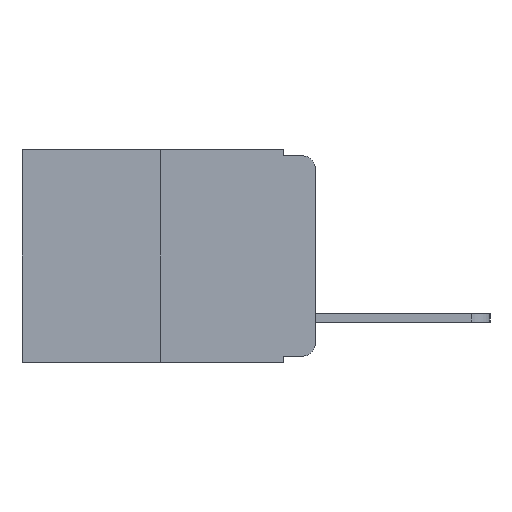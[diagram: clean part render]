
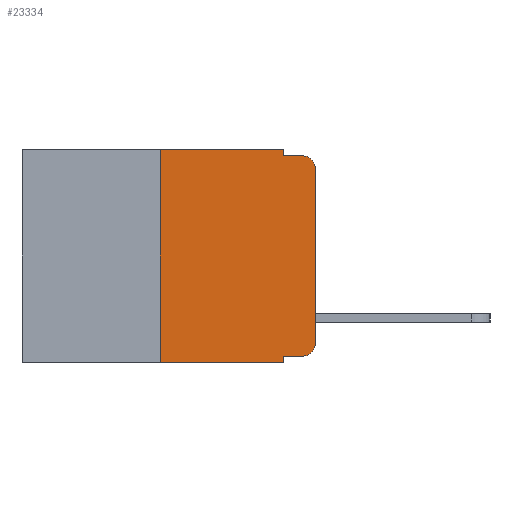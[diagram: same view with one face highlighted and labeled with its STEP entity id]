
A CAD part, left-side view. The second image highlights one B-rep face of the part: STEP entity #23334.
In plain terms, the highlighted planar face has unit normal (-1, 0, 0).
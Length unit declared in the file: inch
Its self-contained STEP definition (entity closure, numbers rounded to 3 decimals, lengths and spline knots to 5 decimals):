
#84 = EDGE_CURVE ( 'NONE', #15799, #23277, #23887, .T. ) ;
#361 = DIRECTION ( 'NONE',  ( 0., 0., -1. ) ) ;
#553 = EDGE_CURVE ( 'NONE', #23277, #15689, #18922, .T. ) ;
#712 = DIRECTION ( 'NONE',  ( 0., -1., 0. ) ) ;
#917 = VERTEX_POINT ( 'NONE', #17587 ) ;
#1067 = DIRECTION ( 'NONE',  ( 0., 0., -1. ) ) ;
#1223 = DIRECTION ( 'NONE',  ( 0., 0., -1. ) ) ;
#2070 = CARTESIAN_POINT ( 'NONE',  ( 0., 0., -0.03 ) ) ;
#2336 = EDGE_CURVE ( 'NONE', #12085, #21058, #13135, .T. ) ;
#2639 = DIRECTION ( 'NONE',  ( -1., 0., 0. ) ) ;
#3029 = CARTESIAN_POINT ( 'NONE',  ( 0., 0.02, -0.313 ) ) ;
#3619 = LINE ( 'NONE', #4112, #12368 ) ;
#4039 = VECTOR ( 'NONE', #19675, 39.37008 ) ;
#4112 = CARTESIAN_POINT ( 'NONE',  ( 0., 0.473, -0.343 ) ) ;
#4740 = VECTOR ( 'NONE', #361, 39.37008 ) ;
#4872 = ORIENTED_EDGE ( 'NONE', *, *, #553, .F. ) ;
#5501 = LINE ( 'NONE', #16483, #14811 ) ;
#6026 = ORIENTED_EDGE ( 'NONE', *, *, #84, .F. ) ;
#6773 = CARTESIAN_POINT ( 'NONE',  ( 0., 0., 0. ) ) ;
#7125 = CARTESIAN_POINT ( 'NONE',  ( 0., 0.02, -0.333 ) ) ;
#7201 = ORIENTED_EDGE ( 'NONE', *, *, #12765, .F. ) ;
#7516 = AXIS2_PLACEMENT_3D ( 'NONE', #23308, #12297, #1067 ) ;
#8140 = CARTESIAN_POINT ( 'NONE',  ( 0., 0.051, -0.01 ) ) ;
#8145 = LINE ( 'NONE', #6773, #17988 ) ;
#8295 = CARTESIAN_POINT ( 'NONE',  ( 0., 0.051, -0.333 ) ) ;
#8583 = CARTESIAN_POINT ( 'NONE',  ( 0., 0.051, 0. ) ) ;
#8944 = DIRECTION ( 'NONE',  ( 0., 0., -1. ) ) ;
#8949 = EDGE_CURVE ( 'NONE', #17417, #12085, #10854, .T. ) ;
#9150 = VECTOR ( 'NONE', #19411, 39.37008 ) ;
#9307 = CARTESIAN_POINT ( 'NONE',  ( 0., 0.051, 0. ) ) ;
#10078 = AXIS2_PLACEMENT_3D ( 'NONE', #3029, #2639, #8944 ) ;
#10107 = ORIENTED_EDGE ( 'NONE', *, *, #21632, .F. ) ;
#10854 = LINE ( 'NONE', #8295, #15743 ) ;
#11007 = DIRECTION ( 'NONE',  ( 0., 0., 1. ) ) ;
#11079 = VERTEX_POINT ( 'NONE', #14723 ) ;
#11113 = VERTEX_POINT ( 'NONE', #2070 ) ;
#11368 = EDGE_CURVE ( 'NONE', #11113, #11079, #21504, .T. ) ;
#11538 = EDGE_LOOP ( 'NONE', ( #20494, #11862, #13038, #4872, #6026, #7201, #18777, #10107, #13610, #12443 ) ) ;
#11862 = ORIENTED_EDGE ( 'NONE', *, *, #11368, .T. ) ;
#12040 = CARTESIAN_POINT ( 'NONE',  ( 0., 0.051, -0.01 ) ) ;
#12085 = VERTEX_POINT ( 'NONE', #7125 ) ;
#12297 = DIRECTION ( 'NONE',  ( -1., 0., 0. ) ) ;
#12368 = VECTOR ( 'NONE', #13474, 39.37008 ) ;
#12426 = DIRECTION ( 'NONE',  ( 1., 0., 0. ) ) ;
#12443 = ORIENTED_EDGE ( 'NONE', *, *, #2336, .T. ) ;
#12765 = EDGE_CURVE ( 'NONE', #17175, #15799, #5501, .T. ) ;
#13038 = ORIENTED_EDGE ( 'NONE', *, *, #16761, .F. ) ;
#13135 = CIRCLE ( 'NONE', #10078, 0.02 ) ;
#13474 = DIRECTION ( 'NONE',  ( 0., -1., 0. ) ) ;
#13610 = ORIENTED_EDGE ( 'NONE', *, *, #8949, .T. ) ;
#13879 = CARTESIAN_POINT ( 'NONE',  ( 0., 0.473, 0. ) ) ;
#14187 = PLANE ( 'NONE',  #20688 ) ;
#14723 = CARTESIAN_POINT ( 'NONE',  ( 0., 0.02, -0.01 ) ) ;
#14811 = VECTOR ( 'NONE', #11007, 39.37008 ) ;
#15689 = VERTEX_POINT ( 'NONE', #12040 ) ;
#15743 = VECTOR ( 'NONE', #21246, 39.37008 ) ;
#15799 = VERTEX_POINT ( 'NONE', #23302 ) ;
#15949 = CARTESIAN_POINT ( 'NONE',  ( 0., 0.473, 0. ) ) ;
#16483 = CARTESIAN_POINT ( 'NONE',  ( 0., 0.25, 0. ) ) ;
#16761 = EDGE_CURVE ( 'NONE', #15689, #11079, #22107, .T. ) ;
#17160 = FACE_OUTER_BOUND ( 'NONE', #11538, .T. ) ;
#17175 = VERTEX_POINT ( 'NONE', #22303 ) ;
#17412 = CARTESIAN_POINT ( 'NONE',  ( 0., 0.051, -0.333 ) ) ;
#17417 = VERTEX_POINT ( 'NONE', #17412 ) ;
#17587 = CARTESIAN_POINT ( 'NONE',  ( 0., 0.051, -0.343 ) ) ;
#17748 = CARTESIAN_POINT ( 'NONE',  ( 0., 0., -0.313 ) ) ;
#17836 = DIRECTION ( 'NONE',  ( 0., 0., 1. ) ) ;
#17912 = EDGE_CURVE ( 'NONE', #17175, #917, #3619, .T. ) ;
#17988 = VECTOR ( 'NONE', #17836, 39.37008 ) ;
#18329 = VECTOR ( 'NONE', #712, 39.37008 ) ;
#18777 = ORIENTED_EDGE ( 'NONE', *, *, #17912, .T. ) ;
#18815 = LINE ( 'NONE', #8583, #4039 ) ;
#18922 = LINE ( 'NONE', #9307, #4740 ) ;
#19411 = DIRECTION ( 'NONE',  ( 0., -1., 0. ) ) ;
#19675 = DIRECTION ( 'NONE',  ( 0., 0., -1. ) ) ;
#20494 = ORIENTED_EDGE ( 'NONE', *, *, #23922, .T. ) ;
#20688 = AXIS2_PLACEMENT_3D ( 'NONE', #15949, #12426, #1223 ) ;
#21058 = VERTEX_POINT ( 'NONE', #17748 ) ;
#21246 = DIRECTION ( 'NONE',  ( 0., -1., 0. ) ) ;
#21445 = CARTESIAN_POINT ( 'NONE',  ( 0., 0.051, 0. ) ) ;
#21504 = CIRCLE ( 'NONE', #7516, 0.02 ) ;
#21632 = EDGE_CURVE ( 'NONE', #17417, #917, #18815, .T. ) ;
#22107 = LINE ( 'NONE', #8140, #18329 ) ;
#22303 = CARTESIAN_POINT ( 'NONE',  ( 0., 0.25, -0.343 ) ) ;
#23277 = VERTEX_POINT ( 'NONE', #21445 ) ;
#23302 = CARTESIAN_POINT ( 'NONE',  ( 0., 0.25, 0. ) ) ;
#23308 = CARTESIAN_POINT ( 'NONE',  ( 0., 0.02, -0.03 ) ) ;
#23334 = ADVANCED_FACE ( 'NONE', ( #17160 ), #14187, .F. ) ;
#23887 = LINE ( 'NONE', #13879, #9150 ) ;
#23922 = EDGE_CURVE ( 'NONE', #21058, #11113, #8145, .T. ) ;
